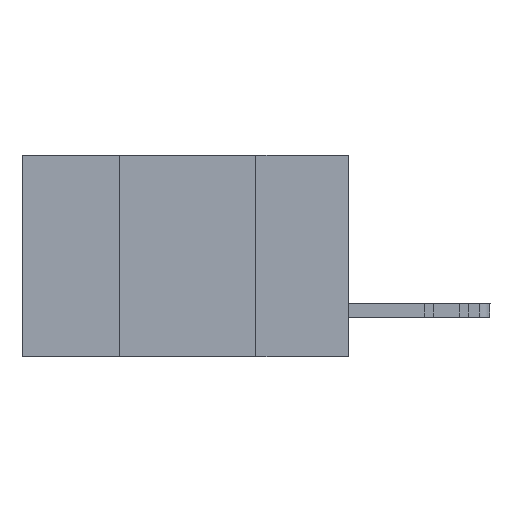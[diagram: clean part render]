
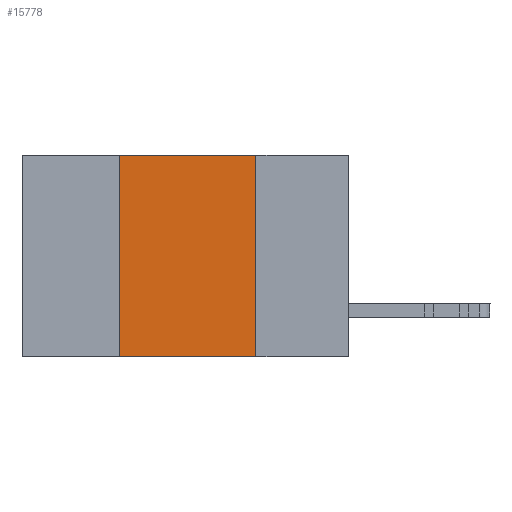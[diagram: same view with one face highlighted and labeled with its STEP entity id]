
A CAD part, left-side view. The second image highlights one B-rep face of the part: STEP entity #15778.
In plain terms, the highlighted planar face has unit normal (-1, 0, 0).
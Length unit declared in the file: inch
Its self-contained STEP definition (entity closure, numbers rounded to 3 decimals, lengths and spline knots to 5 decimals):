
#880 = EDGE_LOOP ( 'NONE', ( #10206, #10820, #940, #6907 ) ) ;
#940 = ORIENTED_EDGE ( 'NONE', *, *, #17435, .F. ) ;
#1186 = VERTEX_POINT ( 'NONE', #22290 ) ;
#2453 = VECTOR ( 'NONE', #21259, 39.37008 ) ;
#4292 = LINE ( 'NONE', #21593, #2453 ) ;
#4302 = VERTEX_POINT ( 'NONE', #5466 ) ;
#4482 = VECTOR ( 'NONE', #20305, 39.37008 ) ;
#4605 = PLANE ( 'NONE',  #12929 ) ;
#4863 = EDGE_CURVE ( 'NONE', #20578, #4302, #4292, .T. ) ;
#5466 = CARTESIAN_POINT ( 'NONE',  ( 0., 0.17, -0.37 ) ) ;
#6115 = EDGE_CURVE ( 'NONE', #1186, #4302, #14766, .T. ) ;
#6907 = ORIENTED_EDGE ( 'NONE', *, *, #4863, .T. ) ;
#7154 = LINE ( 'NONE', #22662, #12249 ) ;
#7819 = LINE ( 'NONE', #12071, #17370 ) ;
#8555 = DIRECTION ( 'NONE',  ( 0., 0., -1. ) ) ;
#10206 = ORIENTED_EDGE ( 'NONE', *, *, #6115, .F. ) ;
#10820 = ORIENTED_EDGE ( 'NONE', *, *, #21756, .F. ) ;
#10961 = FACE_OUTER_BOUND ( 'NONE', #880, .T. ) ;
#12071 = CARTESIAN_POINT ( 'NONE',  ( 0., 0.6, 0. ) ) ;
#12249 = VECTOR ( 'NONE', #17072, 39.37008 ) ;
#12929 = AXIS2_PLACEMENT_3D ( 'NONE', #18038, #19908, #8555 ) ;
#13952 = CARTESIAN_POINT ( 'NONE',  ( 0., 0.42, 0. ) ) ;
#14013 = DIRECTION ( 'NONE',  ( 0., -1., 0. ) ) ;
#14766 = LINE ( 'NONE', #20148, #4482 ) ;
#15087 = VERTEX_POINT ( 'NONE', #13952 ) ;
#15778 = ADVANCED_FACE ( 'NONE', ( #10961 ), #4605, .F. ) ;
#16771 = CARTESIAN_POINT ( 'NONE',  ( 0., 0.42, -0.37 ) ) ;
#17072 = DIRECTION ( 'NONE',  ( 0., 0., 1. ) ) ;
#17370 = VECTOR ( 'NONE', #14013, 39.37008 ) ;
#17435 = EDGE_CURVE ( 'NONE', #20578, #15087, #7154, .T. ) ;
#18038 = CARTESIAN_POINT ( 'NONE',  ( 0., 0.6, 0. ) ) ;
#19908 = DIRECTION ( 'NONE',  ( 1., 0., 0. ) ) ;
#20148 = CARTESIAN_POINT ( 'NONE',  ( 0., 0.17, -0.37 ) ) ;
#20305 = DIRECTION ( 'NONE',  ( 0., 0., -1. ) ) ;
#20578 = VERTEX_POINT ( 'NONE', #16771 ) ;
#21259 = DIRECTION ( 'NONE',  ( 0., -1., 0. ) ) ;
#21593 = CARTESIAN_POINT ( 'NONE',  ( 0., 0.6, -0.37 ) ) ;
#21756 = EDGE_CURVE ( 'NONE', #15087, #1186, #7819, .T. ) ;
#22290 = CARTESIAN_POINT ( 'NONE',  ( 0., 0.17, 0. ) ) ;
#22662 = CARTESIAN_POINT ( 'NONE',  ( 0., 0.42, -0.37 ) ) ;
